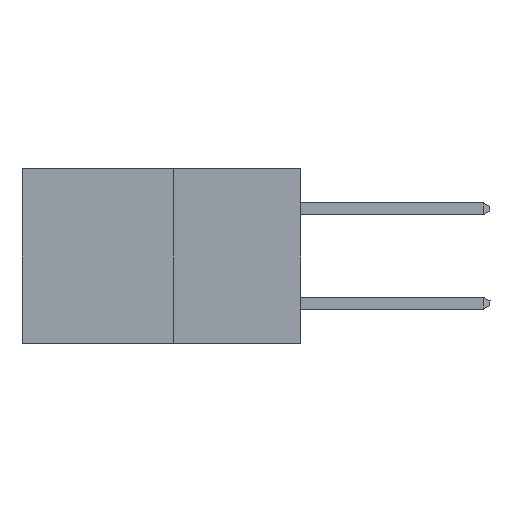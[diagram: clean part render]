
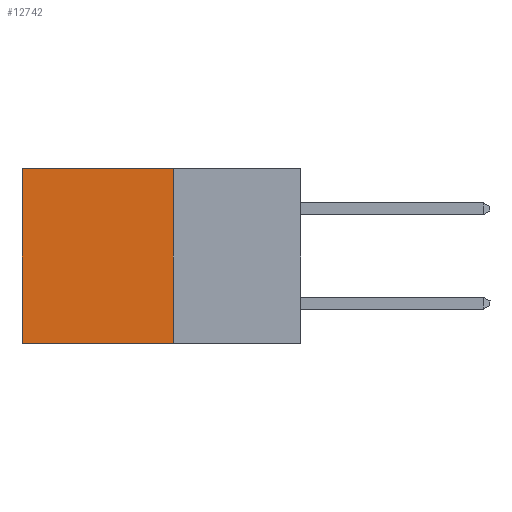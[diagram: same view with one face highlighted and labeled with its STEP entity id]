
A CAD part, left-side view. The second image highlights one B-rep face of the part: STEP entity #12742.
In plain terms, the highlighted planar face has unit normal (-1, 0, 0).
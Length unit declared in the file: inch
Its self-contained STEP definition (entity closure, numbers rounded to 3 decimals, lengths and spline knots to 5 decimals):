
#2491 = CARTESIAN_POINT ( 'NONE',  ( 0.277, 0.27, 0. ) ) ;
#3152 = VECTOR ( 'NONE', #5074, 39.37008 ) ;
#3956 = ORIENTED_EDGE ( 'NONE', *, *, #19111, .T. ) ;
#4365 = AXIS2_PLACEMENT_3D ( 'NONE', #15411, #22864, #7985 ) ;
#5074 = DIRECTION ( 'NONE',  ( 0., 1., 0. ) ) ;
#7985 = DIRECTION ( 'NONE',  ( 0., 0., -1. ) ) ;
#8182 = EDGE_LOOP ( 'NONE', ( #27445, #21249, #20488, #3956 ) ) ;
#8383 = EDGE_CURVE ( 'NONE', #16445, #30256, #32146, .T. ) ;
#10600 = DIRECTION ( 'NONE',  ( 0., 0., -1. ) ) ;
#10924 = CARTESIAN_POINT ( 'NONE',  ( 0.277, 0.59, 0. ) ) ;
#10996 = LINE ( 'NONE', #29774, #16845 ) ;
#12742 = ADVANCED_FACE ( 'NONE', ( #13290 ), #22764, .F. ) ;
#13290 = FACE_OUTER_BOUND ( 'NONE', #8182, .T. ) ;
#13424 = VERTEX_POINT ( 'NONE', #10924 ) ;
#15411 = CARTESIAN_POINT ( 'NONE',  ( 0.277, 0.27, -0.37 ) ) ;
#16445 = VERTEX_POINT ( 'NONE', #16498 ) ;
#16498 = CARTESIAN_POINT ( 'NONE',  ( 0.277, 0.27, -0.37 ) ) ;
#16845 = VECTOR ( 'NONE', #10600, 39.37008 ) ;
#18004 = DIRECTION ( 'NONE',  ( 0., 1., 0. ) ) ;
#19111 = EDGE_CURVE ( 'NONE', #21397, #13424, #29588, .T. ) ;
#19330 = CARTESIAN_POINT ( 'NONE',  ( 0.277, 0.59, -0.37 ) ) ;
#20488 = ORIENTED_EDGE ( 'NONE', *, *, #22972, .F. ) ;
#21249 = ORIENTED_EDGE ( 'NONE', *, *, #8383, .F. ) ;
#21397 = VERTEX_POINT ( 'NONE', #27929 ) ;
#22764 = PLANE ( 'NONE',  #4365 ) ;
#22864 = DIRECTION ( 'NONE',  ( 1., 0., 0. ) ) ;
#22972 = EDGE_CURVE ( 'NONE', #21397, #16445, #10996, .T. ) ;
#25642 = VECTOR ( 'NONE', #18004, 39.37008 ) ;
#25849 = LINE ( 'NONE', #29574, #31572 ) ;
#27445 = ORIENTED_EDGE ( 'NONE', *, *, #31080, .T. ) ;
#27929 = CARTESIAN_POINT ( 'NONE',  ( 0.277, 0.27, 0. ) ) ;
#29574 = CARTESIAN_POINT ( 'NONE',  ( 0.277, 0.59, -0.37 ) ) ;
#29588 = LINE ( 'NONE', #2491, #3152 ) ;
#29774 = CARTESIAN_POINT ( 'NONE',  ( 0.277, 0.27, -0.37 ) ) ;
#30236 = CARTESIAN_POINT ( 'NONE',  ( 0.277, 0.27, -0.37 ) ) ;
#30256 = VERTEX_POINT ( 'NONE', #19330 ) ;
#31080 = EDGE_CURVE ( 'NONE', #13424, #30256, #25849, .T. ) ;
#31572 = VECTOR ( 'NONE', #32055, 39.37008 ) ;
#32055 = DIRECTION ( 'NONE',  ( 0., 0., -1. ) ) ;
#32146 = LINE ( 'NONE', #30236, #25642 ) ;
